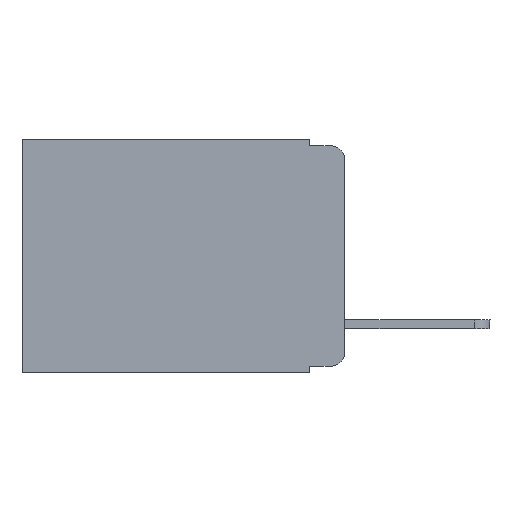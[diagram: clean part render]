
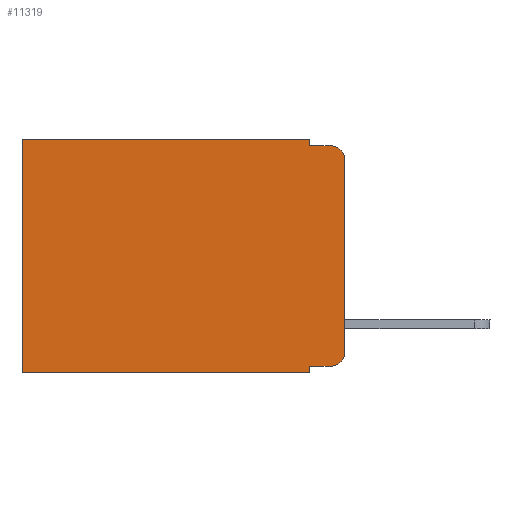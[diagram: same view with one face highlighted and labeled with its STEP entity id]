
A CAD part, left-side view. The second image highlights one B-rep face of the part: STEP entity #11319.
In plain terms, the highlighted planar face has unit normal (-1, 0, 0).
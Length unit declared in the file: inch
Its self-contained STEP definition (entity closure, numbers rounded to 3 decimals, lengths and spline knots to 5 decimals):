
#445 = PLANE ( 'NONE',  #18388 ) ;
#557 = DIRECTION ( 'NONE',  ( -1., 0., 0. ) ) ;
#669 = DIRECTION ( 'NONE',  ( 0., 0., -1. ) ) ;
#690 = CARTESIAN_POINT ( 'NONE',  ( 0.298, 0., -0.343 ) ) ;
#924 = CARTESIAN_POINT ( 'NONE',  ( 0.298, 0.051, -0.343 ) ) ;
#980 = DIRECTION ( 'NONE',  ( 0., 0., -1. ) ) ;
#1314 = CARTESIAN_POINT ( 'NONE',  ( 0.298, 0.02, -0.333 ) ) ;
#1905 = VECTOR ( 'NONE', #3827, 39.37008 ) ;
#2316 = CARTESIAN_POINT ( 'NONE',  ( 0.298, 0., -0.03 ) ) ;
#2948 = CARTESIAN_POINT ( 'NONE',  ( 0.298, 0., -0.313 ) ) ;
#3463 = CARTESIAN_POINT ( 'NONE',  ( 0.298, 0.051, -0.333 ) ) ;
#3503 = VERTEX_POINT ( 'NONE', #2948 ) ;
#3606 = VECTOR ( 'NONE', #19201, 39.37008 ) ;
#3827 = DIRECTION ( 'NONE',  ( 0., 1., 0. ) ) ;
#3845 = VERTEX_POINT ( 'NONE', #20776 ) ;
#4213 = DIRECTION ( 'NONE',  ( 0., 1., 0. ) ) ;
#4271 = DIRECTION ( 'NONE',  ( 0., 0., -1. ) ) ;
#4358 = ORIENTED_EDGE ( 'NONE', *, *, #16401, .F. ) ;
#4632 = CARTESIAN_POINT ( 'NONE',  ( 0.298, 0., 0. ) ) ;
#4758 = EDGE_CURVE ( 'NONE', #20951, #3845, #10754, .T. ) ;
#5342 = VERTEX_POINT ( 'NONE', #12967 ) ;
#5452 = EDGE_CURVE ( 'NONE', #18774, #3503, #11330, .T. ) ;
#5992 = VERTEX_POINT ( 'NONE', #1314 ) ;
#7680 = CARTESIAN_POINT ( 'NONE',  ( 0.298, 0.02, -0.03 ) ) ;
#7684 = LINE ( 'NONE', #12615, #1905 ) ;
#8141 = LINE ( 'NONE', #19064, #13910 ) ;
#8587 = VECTOR ( 'NONE', #14266, 39.37008 ) ;
#8785 = LINE ( 'NONE', #12535, #10861 ) ;
#8904 = CARTESIAN_POINT ( 'NONE',  ( 0.298, 0.473, 0. ) ) ;
#9104 = CARTESIAN_POINT ( 'NONE',  ( 0.298, 0.051, 0. ) ) ;
#9132 = DIRECTION ( 'NONE',  ( 1., 0., 0. ) ) ;
#9220 = EDGE_LOOP ( 'NONE', ( #14028, #21625, #18442, #4358, #9548, #19178, #14288, #15529, #17371, #19209 ) ) ;
#9540 = EDGE_CURVE ( 'NONE', #14176, #15312, #12312, .T. ) ;
#9548 = ORIENTED_EDGE ( 'NONE', *, *, #21083, .T. ) ;
#9722 = LINE ( 'NONE', #690, #16407 ) ;
#10010 = EDGE_CURVE ( 'NONE', #11792, #14310, #15484, .T. ) ;
#10286 = CARTESIAN_POINT ( 'NONE',  ( 0.298, 0.473, 0. ) ) ;
#10754 = LINE ( 'NONE', #8904, #19430 ) ;
#10839 = AXIS2_PLACEMENT_3D ( 'NONE', #7680, #13204, #4271 ) ;
#10861 = VECTOR ( 'NONE', #10990, 39.37008 ) ;
#10990 = DIRECTION ( 'NONE',  ( 0., -1., 0. ) ) ;
#11319 = ADVANCED_FACE ( 'NONE', ( #12531 ), #445, .F. ) ;
#11330 = LINE ( 'NONE', #4632, #3606 ) ;
#11792 = VERTEX_POINT ( 'NONE', #3463 ) ;
#12312 = LINE ( 'NONE', #20893, #16805 ) ;
#12531 = FACE_OUTER_BOUND ( 'NONE', #9220, .T. ) ;
#12535 = CARTESIAN_POINT ( 'NONE',  ( 0.298, 0.051, -0.333 ) ) ;
#12539 = DIRECTION ( 'NONE',  ( 0., 0., -1. ) ) ;
#12615 = CARTESIAN_POINT ( 'NONE',  ( 0.298, 0., 0. ) ) ;
#12784 = EDGE_CURVE ( 'NONE', #14310, #3845, #9722, .T. ) ;
#12967 = CARTESIAN_POINT ( 'NONE',  ( 0.298, 0.051, 0. ) ) ;
#12984 = CARTESIAN_POINT ( 'NONE',  ( 0.298, 0.02, -0.313 ) ) ;
#13204 = DIRECTION ( 'NONE',  ( -1., 0., 0. ) ) ;
#13910 = VECTOR ( 'NONE', #980, 39.37008 ) ;
#14028 = ORIENTED_EDGE ( 'NONE', *, *, #5452, .F. ) ;
#14076 = DIRECTION ( 'NONE',  ( 0., -1., 0. ) ) ;
#14176 = VERTEX_POINT ( 'NONE', #20056 ) ;
#14266 = DIRECTION ( 'NONE',  ( 0., 0., -1. ) ) ;
#14288 = ORIENTED_EDGE ( 'NONE', *, *, #12784, .F. ) ;
#14310 = VERTEX_POINT ( 'NONE', #924 ) ;
#14404 = DIRECTION ( 'NONE',  ( 0., 0., -1. ) ) ;
#14689 = EDGE_CURVE ( 'NONE', #5992, #3503, #17268, .T. ) ;
#15072 = EDGE_CURVE ( 'NONE', #18774, #15312, #22865, .T. ) ;
#15312 = VERTEX_POINT ( 'NONE', #21718 ) ;
#15484 = LINE ( 'NONE', #9104, #8587 ) ;
#15529 = ORIENTED_EDGE ( 'NONE', *, *, #10010, .F. ) ;
#15718 = EDGE_CURVE ( 'NONE', #11792, #5992, #8785, .T. ) ;
#16401 = EDGE_CURVE ( 'NONE', #5342, #14176, #8141, .T. ) ;
#16407 = VECTOR ( 'NONE', #4213, 39.37008 ) ;
#16805 = VECTOR ( 'NONE', #14076, 39.37008 ) ;
#17268 = CIRCLE ( 'NONE', #18399, 0.02 ) ;
#17371 = ORIENTED_EDGE ( 'NONE', *, *, #15718, .T. ) ;
#18388 = AXIS2_PLACEMENT_3D ( 'NONE', #19691, #9132, #14404 ) ;
#18399 = AXIS2_PLACEMENT_3D ( 'NONE', #12984, #557, #669 ) ;
#18442 = ORIENTED_EDGE ( 'NONE', *, *, #9540, .F. ) ;
#18774 = VERTEX_POINT ( 'NONE', #2316 ) ;
#19064 = CARTESIAN_POINT ( 'NONE',  ( 0.298, 0.051, 0. ) ) ;
#19178 = ORIENTED_EDGE ( 'NONE', *, *, #4758, .T. ) ;
#19201 = DIRECTION ( 'NONE',  ( 0., 0., -1. ) ) ;
#19209 = ORIENTED_EDGE ( 'NONE', *, *, #14689, .T. ) ;
#19430 = VECTOR ( 'NONE', #12539, 39.37008 ) ;
#19691 = CARTESIAN_POINT ( 'NONE',  ( 0.298, 0., 0. ) ) ;
#20056 = CARTESIAN_POINT ( 'NONE',  ( 0.298, 0.051, -0.01 ) ) ;
#20776 = CARTESIAN_POINT ( 'NONE',  ( 0.298, 0.473, -0.343 ) ) ;
#20893 = CARTESIAN_POINT ( 'NONE',  ( 0.298, 0.051, -0.01 ) ) ;
#20951 = VERTEX_POINT ( 'NONE', #10286 ) ;
#21083 = EDGE_CURVE ( 'NONE', #5342, #20951, #7684, .T. ) ;
#21625 = ORIENTED_EDGE ( 'NONE', *, *, #15072, .T. ) ;
#21718 = CARTESIAN_POINT ( 'NONE',  ( 0.298, 0.02, -0.01 ) ) ;
#22865 = CIRCLE ( 'NONE', #10839, 0.02 ) ;
